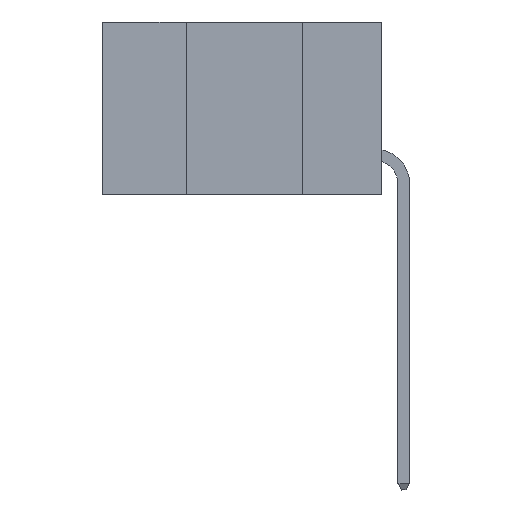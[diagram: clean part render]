
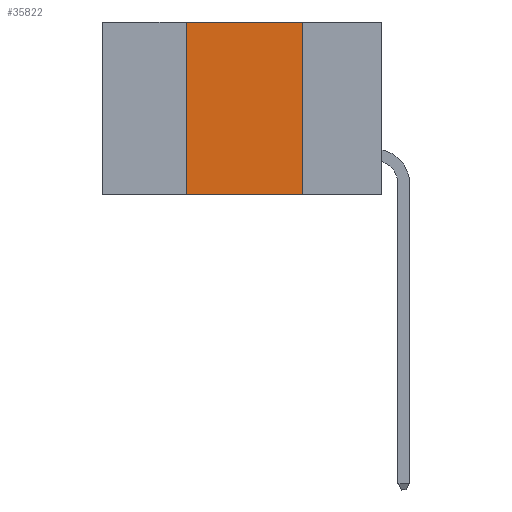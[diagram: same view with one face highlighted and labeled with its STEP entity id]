
A CAD part, left-side view. The second image highlights one B-rep face of the part: STEP entity #35822.
In plain terms, the highlighted planar face has unit normal (-1, 0, 0).
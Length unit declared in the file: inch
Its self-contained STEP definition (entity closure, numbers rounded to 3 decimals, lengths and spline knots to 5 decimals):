
#172 = AXIS2_PLACEMENT_3D ( 'NONE', #31927, #6123, #26005 ) ;
#352 = VERTEX_POINT ( 'NONE', #22273 ) ;
#837 = VERTEX_POINT ( 'NONE', #27443 ) ;
#891 = EDGE_CURVE ( 'NONE', #34879, #352, #35961, .T. ) ;
#3230 = PLANE ( 'NONE',  #172 ) ;
#3573 = ORIENTED_EDGE ( 'NONE', *, *, #22376, .F. ) ;
#4559 = VERTEX_POINT ( 'NONE', #23007 ) ;
#5575 = CARTESIAN_POINT ( 'NONE',  ( 0., 0.42, 0. ) ) ;
#6005 = EDGE_LOOP ( 'NONE', ( #6740, #17000, #3573, #13000 ) ) ;
#6123 = DIRECTION ( 'NONE',  ( 1., 0., 0. ) ) ;
#6740 = ORIENTED_EDGE ( 'NONE', *, *, #891, .F. ) ;
#6816 = CARTESIAN_POINT ( 'NONE',  ( 0., 0.17, 0. ) ) ;
#7635 = DIRECTION ( 'NONE',  ( 0., -1., 0. ) ) ;
#8432 = VECTOR ( 'NONE', #37045, 39.37008 ) ;
#8770 = FACE_OUTER_BOUND ( 'NONE', #6005, .T. ) ;
#10756 = VECTOR ( 'NONE', #7635, 39.37008 ) ;
#13000 = ORIENTED_EDGE ( 'NONE', *, *, #37157, .T. ) ;
#13321 = CARTESIAN_POINT ( 'NONE',  ( 0., 0.17, 0. ) ) ;
#15553 = EDGE_CURVE ( 'NONE', #4559, #34879, #28024, .T. ) ;
#15681 = DIRECTION ( 'NONE',  ( 0., 0., -1. ) ) ;
#17000 = ORIENTED_EDGE ( 'NONE', *, *, #15553, .F. ) ;
#17161 = VECTOR ( 'NONE', #29678, 39.37008 ) ;
#22273 = CARTESIAN_POINT ( 'NONE',  ( 0., 0.17, -0.37 ) ) ;
#22376 = EDGE_CURVE ( 'NONE', #837, #4559, #33220, .T. ) ;
#22412 = LINE ( 'NONE', #30542, #10756 ) ;
#23007 = CARTESIAN_POINT ( 'NONE',  ( 0., 0.42, 0. ) ) ;
#23863 = CARTESIAN_POINT ( 'NONE',  ( 0., 0.6, 0. ) ) ;
#26005 = DIRECTION ( 'NONE',  ( 0., 0., -1. ) ) ;
#27443 = CARTESIAN_POINT ( 'NONE',  ( 0., 0.42, -0.37 ) ) ;
#28024 = LINE ( 'NONE', #23863, #17161 ) ;
#29678 = DIRECTION ( 'NONE',  ( 0., -1., 0. ) ) ;
#30542 = CARTESIAN_POINT ( 'NONE',  ( 0., 0.6, -0.37 ) ) ;
#31927 = CARTESIAN_POINT ( 'NONE',  ( 0., 0.6, 0. ) ) ;
#33220 = LINE ( 'NONE', #5575, #8432 ) ;
#33260 = VECTOR ( 'NONE', #15681, 39.37008 ) ;
#34879 = VERTEX_POINT ( 'NONE', #6816 ) ;
#35822 = ADVANCED_FACE ( 'NONE', ( #8770 ), #3230, .F. ) ;
#35961 = LINE ( 'NONE', #13321, #33260 ) ;
#37045 = DIRECTION ( 'NONE',  ( 0., 0., 1. ) ) ;
#37157 = EDGE_CURVE ( 'NONE', #837, #352, #22412, .T. ) ;
